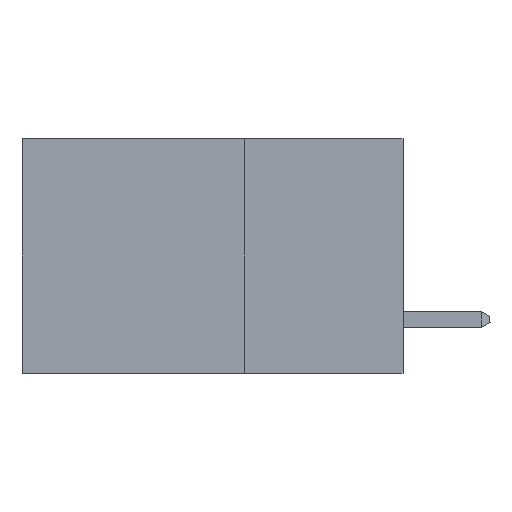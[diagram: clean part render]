
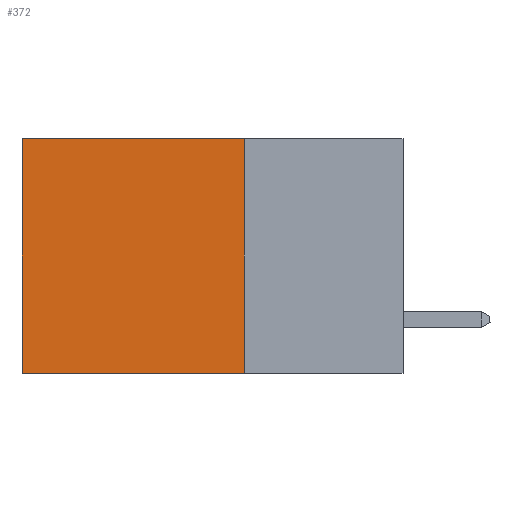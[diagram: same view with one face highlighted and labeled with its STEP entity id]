
A CAD part, left-side view. The second image highlights one B-rep face of the part: STEP entity #372.
In plain terms, the highlighted planar face has unit normal (-1, 0, 0).
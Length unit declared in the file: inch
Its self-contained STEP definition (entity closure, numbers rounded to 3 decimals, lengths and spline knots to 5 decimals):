
#372 = ADVANCED_FACE ( 'NONE', ( #7391 ), #5432, .F. ) ;
#446 = VERTEX_POINT ( 'NONE', #15812 ) ;
#723 = CARTESIAN_POINT ( 'NONE',  ( 0.2875, 0.6, 0. ) ) ;
#1459 = CARTESIAN_POINT ( 'NONE',  ( 0.2875, 0.25, 0. ) ) ;
#1613 = CARTESIAN_POINT ( 'NONE',  ( 0.2875, 0.25, 0. ) ) ;
#1722 = DIRECTION ( 'NONE',  ( 0., 0., -1. ) ) ;
#2183 = VERTEX_POINT ( 'NONE', #1459 ) ;
#2211 = LINE ( 'NONE', #5136, #5527 ) ;
#2536 = CARTESIAN_POINT ( 'NONE',  ( 0.2875, 0.25, -0.37 ) ) ;
#3084 = EDGE_CURVE ( 'NONE', #2183, #8213, #13083, .T. ) ;
#4257 = ORIENTED_EDGE ( 'NONE', *, *, #3084, .F. ) ;
#4623 = VECTOR ( 'NONE', #5842, 39.37008 ) ;
#5136 = CARTESIAN_POINT ( 'NONE',  ( 0.2875, 0.25, 0. ) ) ;
#5272 = VECTOR ( 'NONE', #7451, 39.37008 ) ;
#5428 = EDGE_CURVE ( 'NONE', #2183, #8466, #2211, .T. ) ;
#5432 = PLANE ( 'NONE',  #8182 ) ;
#5527 = VECTOR ( 'NONE', #12711, 39.37008 ) ;
#5637 = ORIENTED_EDGE ( 'NONE', *, *, #6817, .F. ) ;
#5668 = LINE ( 'NONE', #11316, #5272 ) ;
#5842 = DIRECTION ( 'NONE',  ( 0., 0., -1. ) ) ;
#6817 = EDGE_CURVE ( 'NONE', #8213, #446, #5668, .T. ) ;
#7391 = FACE_OUTER_BOUND ( 'NONE', #15475, .T. ) ;
#7451 = DIRECTION ( 'NONE',  ( 0., 1., 0. ) ) ;
#7969 = DIRECTION ( 'NONE',  ( 1., 0., 0. ) ) ;
#8182 = AXIS2_PLACEMENT_3D ( 'NONE', #1613, #7969, #1722 ) ;
#8213 = VERTEX_POINT ( 'NONE', #2536 ) ;
#8323 = VECTOR ( 'NONE', #8423, 39.37008 ) ;
#8423 = DIRECTION ( 'NONE',  ( 0., 0., -1. ) ) ;
#8466 = VERTEX_POINT ( 'NONE', #11635 ) ;
#8699 = EDGE_CURVE ( 'NONE', #8466, #446, #10327, .T. ) ;
#10180 = ORIENTED_EDGE ( 'NONE', *, *, #5428, .T. ) ;
#10327 = LINE ( 'NONE', #723, #4623 ) ;
#10561 = ORIENTED_EDGE ( 'NONE', *, *, #8699, .T. ) ;
#11316 = CARTESIAN_POINT ( 'NONE',  ( 0.2875, 0.25, -0.37 ) ) ;
#11635 = CARTESIAN_POINT ( 'NONE',  ( 0.2875, 0.6, 0. ) ) ;
#11900 = CARTESIAN_POINT ( 'NONE',  ( 0.2875, 0.25, 0. ) ) ;
#12711 = DIRECTION ( 'NONE',  ( 0., 1., 0. ) ) ;
#13083 = LINE ( 'NONE', #11900, #8323 ) ;
#15475 = EDGE_LOOP ( 'NONE', ( #10561, #5637, #4257, #10180 ) ) ;
#15812 = CARTESIAN_POINT ( 'NONE',  ( 0.2875, 0.6, -0.37 ) ) ;
